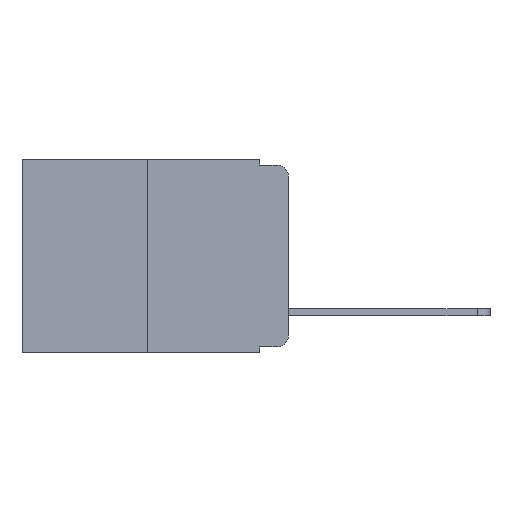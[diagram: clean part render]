
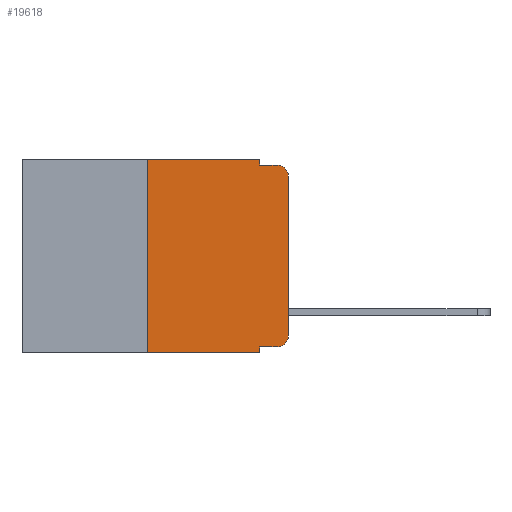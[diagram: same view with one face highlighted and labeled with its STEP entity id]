
A CAD part, left-side view. The second image highlights one B-rep face of the part: STEP entity #19618.
In plain terms, the highlighted planar face has unit normal (-1, 0, 0).
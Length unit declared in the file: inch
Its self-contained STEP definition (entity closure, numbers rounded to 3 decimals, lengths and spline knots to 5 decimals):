
#635 = DIRECTION ( 'NONE',  ( 0., 0., -1. ) ) ;
#686 = CIRCLE ( 'NONE', #12774, 0.02 ) ;
#796 = AXIS2_PLACEMENT_3D ( 'NONE', #12229, #15463, #5539 ) ;
#1143 = LINE ( 'NONE', #11641, #21256 ) ;
#1265 = CARTESIAN_POINT ( 'NONE',  ( 0., 0., -0.03 ) ) ;
#1281 = DIRECTION ( 'NONE',  ( 0., 0., 1. ) ) ;
#1469 = DIRECTION ( 'NONE',  ( 0., 0., -1. ) ) ;
#1760 = CARTESIAN_POINT ( 'NONE',  ( 0., 0.051, -0.343 ) ) ;
#1956 = LINE ( 'NONE', #21266, #5554 ) ;
#1982 = CARTESIAN_POINT ( 'NONE',  ( 0., 0.051, -0.01 ) ) ;
#2839 = DIRECTION ( 'NONE',  ( 0., 0., -1. ) ) ;
#3267 = VECTOR ( 'NONE', #3526, 39.37008 ) ;
#3526 = DIRECTION ( 'NONE',  ( 0., -1., 0. ) ) ;
#4136 = LINE ( 'NONE', #1982, #16398 ) ;
#4293 = CARTESIAN_POINT ( 'NONE',  ( 0., 0.473, -0.343 ) ) ;
#4329 = VERTEX_POINT ( 'NONE', #1760 ) ;
#4959 = VERTEX_POINT ( 'NONE', #21509 ) ;
#5479 = VERTEX_POINT ( 'NONE', #16163 ) ;
#5539 = DIRECTION ( 'NONE',  ( 0., 0., -1. ) ) ;
#5554 = VECTOR ( 'NONE', #1281, 39.37008 ) ;
#6019 = VECTOR ( 'NONE', #2839, 39.37008 ) ;
#6404 = AXIS2_PLACEMENT_3D ( 'NONE', #21419, #11747, #1469 ) ;
#6564 = LINE ( 'NONE', #7975, #6019 ) ;
#6814 = DIRECTION ( 'NONE',  ( 0., -1., 0. ) ) ;
#7252 = VECTOR ( 'NONE', #6814, 39.37008 ) ;
#7305 = LINE ( 'NONE', #16940, #3267 ) ;
#7322 = EDGE_CURVE ( 'NONE', #13150, #5479, #686, .T. ) ;
#7717 = VERTEX_POINT ( 'NONE', #19989 ) ;
#7782 = ORIENTED_EDGE ( 'NONE', *, *, #16155, .T. ) ;
#7975 = CARTESIAN_POINT ( 'NONE',  ( 0., 0.051, 0. ) ) ;
#8146 = CARTESIAN_POINT ( 'NONE',  ( 0., 0.25, 0. ) ) ;
#8444 = EDGE_CURVE ( 'NONE', #18698, #13150, #7305, .T. ) ;
#8541 = LINE ( 'NONE', #18677, #21525 ) ;
#8834 = DIRECTION ( 'NONE',  ( 0., 0., -1. ) ) ;
#8957 = VERTEX_POINT ( 'NONE', #1265 ) ;
#9073 = ORIENTED_EDGE ( 'NONE', *, *, #7322, .T. ) ;
#9414 = EDGE_CURVE ( 'NONE', #19298, #20753, #20288, .T. ) ;
#9556 = EDGE_CURVE ( 'NONE', #18698, #4329, #8541, .T. ) ;
#10373 = ORIENTED_EDGE ( 'NONE', *, *, #10650, .F. ) ;
#10650 = EDGE_CURVE ( 'NONE', #7717, #19298, #1956, .T. ) ;
#11025 = DIRECTION ( 'NONE',  ( -1., 0., 0. ) ) ;
#11641 = CARTESIAN_POINT ( 'NONE',  ( 0., 0., 0. ) ) ;
#11747 = DIRECTION ( 'NONE',  ( -1., 0., 0. ) ) ;
#11804 = EDGE_CURVE ( 'NONE', #20753, #4959, #6564, .T. ) ;
#12224 = DIRECTION ( 'NONE',  ( 0., -1., 0. ) ) ;
#12229 = CARTESIAN_POINT ( 'NONE',  ( 0., 0.473, 0. ) ) ;
#12406 = VECTOR ( 'NONE', #14348, 39.37008 ) ;
#12489 = ORIENTED_EDGE ( 'NONE', *, *, #9556, .F. ) ;
#12774 = AXIS2_PLACEMENT_3D ( 'NONE', #20749, #11025, #635 ) ;
#13150 = VERTEX_POINT ( 'NONE', #20144 ) ;
#13767 = ORIENTED_EDGE ( 'NONE', *, *, #11804, .F. ) ;
#13870 = PLANE ( 'NONE',  #796 ) ;
#14003 = EDGE_CURVE ( 'NONE', #4959, #20102, #4136, .T. ) ;
#14270 = ORIENTED_EDGE ( 'NONE', *, *, #9414, .F. ) ;
#14348 = DIRECTION ( 'NONE',  ( 0., -1., 0. ) ) ;
#14856 = DIRECTION ( 'NONE',  ( 0., 0., 1. ) ) ;
#15073 = EDGE_CURVE ( 'NONE', #8957, #20102, #16589, .T. ) ;
#15463 = DIRECTION ( 'NONE',  ( 1., 0., 0. ) ) ;
#15767 = ORIENTED_EDGE ( 'NONE', *, *, #19020, .T. ) ;
#16155 = EDGE_CURVE ( 'NONE', #5479, #8957, #1143, .T. ) ;
#16163 = CARTESIAN_POINT ( 'NONE',  ( 0., 0., -0.313 ) ) ;
#16398 = VECTOR ( 'NONE', #12224, 39.37008 ) ;
#16589 = CIRCLE ( 'NONE', #6404, 0.02 ) ;
#16593 = CARTESIAN_POINT ( 'NONE',  ( 0., 0.02, -0.01 ) ) ;
#16718 = LINE ( 'NONE', #4293, #12406 ) ;
#16940 = CARTESIAN_POINT ( 'NONE',  ( 0., 0.051, -0.333 ) ) ;
#17549 = ORIENTED_EDGE ( 'NONE', *, *, #15073, .T. ) ;
#17969 = FACE_OUTER_BOUND ( 'NONE', #20052, .T. ) ;
#18334 = CARTESIAN_POINT ( 'NONE',  ( 0., 0.051, -0.333 ) ) ;
#18339 = CARTESIAN_POINT ( 'NONE',  ( 0., 0.473, 0. ) ) ;
#18677 = CARTESIAN_POINT ( 'NONE',  ( 0., 0.051, 0. ) ) ;
#18698 = VERTEX_POINT ( 'NONE', #18334 ) ;
#19020 = EDGE_CURVE ( 'NONE', #7717, #4329, #16718, .T. ) ;
#19298 = VERTEX_POINT ( 'NONE', #8146 ) ;
#19618 = ADVANCED_FACE ( 'NONE', ( #17969 ), #13870, .F. ) ;
#19989 = CARTESIAN_POINT ( 'NONE',  ( 0., 0.25, -0.343 ) ) ;
#20025 = CARTESIAN_POINT ( 'NONE',  ( 0., 0.051, 0. ) ) ;
#20052 = EDGE_LOOP ( 'NONE', ( #7782, #17549, #21789, #13767, #14270, #10373, #15767, #12489, #21555, #9073 ) ) ;
#20102 = VERTEX_POINT ( 'NONE', #16593 ) ;
#20144 = CARTESIAN_POINT ( 'NONE',  ( 0., 0.02, -0.333 ) ) ;
#20288 = LINE ( 'NONE', #18339, #7252 ) ;
#20749 = CARTESIAN_POINT ( 'NONE',  ( 0., 0.02, -0.313 ) ) ;
#20753 = VERTEX_POINT ( 'NONE', #20025 ) ;
#21256 = VECTOR ( 'NONE', #14856, 39.37008 ) ;
#21266 = CARTESIAN_POINT ( 'NONE',  ( 0., 0.25, 0. ) ) ;
#21419 = CARTESIAN_POINT ( 'NONE',  ( 0., 0.02, -0.03 ) ) ;
#21509 = CARTESIAN_POINT ( 'NONE',  ( 0., 0.051, -0.01 ) ) ;
#21525 = VECTOR ( 'NONE', #8834, 39.37008 ) ;
#21555 = ORIENTED_EDGE ( 'NONE', *, *, #8444, .T. ) ;
#21789 = ORIENTED_EDGE ( 'NONE', *, *, #14003, .F. ) ;
